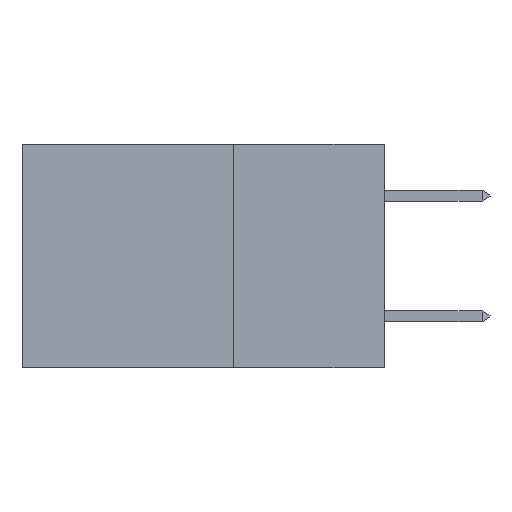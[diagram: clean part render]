
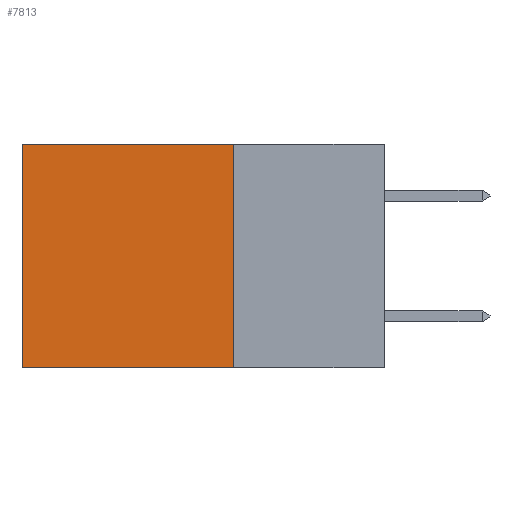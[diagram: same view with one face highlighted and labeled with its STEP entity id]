
A CAD part, left-side view. The second image highlights one B-rep face of the part: STEP entity #7813.
In plain terms, the highlighted planar face has unit normal (-1, 0, 0).
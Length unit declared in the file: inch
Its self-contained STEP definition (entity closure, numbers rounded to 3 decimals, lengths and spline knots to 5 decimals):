
#55 = VECTOR ( 'NONE', #8154, 39.37008 ) ;
#814 = EDGE_CURVE ( 'NONE', #9395, #15665, #13085, .T. ) ;
#1489 = ORIENTED_EDGE ( 'NONE', *, *, #814, .F. ) ;
#1760 = ORIENTED_EDGE ( 'NONE', *, *, #6386, .F. ) ;
#2906 = CARTESIAN_POINT ( 'NONE',  ( 0.2875, 0.25, 0. ) ) ;
#2936 = CARTESIAN_POINT ( 'NONE',  ( 0.2875, 0.25, 0. ) ) ;
#4235 = FACE_OUTER_BOUND ( 'NONE', #13283, .T. ) ;
#4544 = EDGE_CURVE ( 'NONE', #9395, #8620, #5394, .T. ) ;
#4994 = VERTEX_POINT ( 'NONE', #5558 ) ;
#5353 = CARTESIAN_POINT ( 'NONE',  ( 0.2875, 0.25, -0.37 ) ) ;
#5394 = LINE ( 'NONE', #11335, #7555 ) ;
#5558 = CARTESIAN_POINT ( 'NONE',  ( 0.2875, 0.6, -0.37 ) ) ;
#6169 = AXIS2_PLACEMENT_3D ( 'NONE', #2906, #8652, #14366 ) ;
#6386 = EDGE_CURVE ( 'NONE', #15665, #4994, #16621, .T. ) ;
#7189 = CARTESIAN_POINT ( 'NONE',  ( 0.2875, 0.6, 0. ) ) ;
#7555 = VECTOR ( 'NONE', #8414, 39.37008 ) ;
#7813 = ADVANCED_FACE ( 'NONE', ( #4235 ), #14451, .F. ) ;
#8154 = DIRECTION ( 'NONE',  ( 0., 0., -1. ) ) ;
#8414 = DIRECTION ( 'NONE',  ( 0., 1., 0. ) ) ;
#8620 = VERTEX_POINT ( 'NONE', #7189 ) ;
#8652 = DIRECTION ( 'NONE',  ( 1., 0., 0. ) ) ;
#9322 = CARTESIAN_POINT ( 'NONE',  ( 0.2875, 0.25, 0. ) ) ;
#9395 = VERTEX_POINT ( 'NONE', #9322 ) ;
#9489 = VECTOR ( 'NONE', #11600, 39.37008 ) ;
#11230 = ORIENTED_EDGE ( 'NONE', *, *, #4544, .T. ) ;
#11335 = CARTESIAN_POINT ( 'NONE',  ( 0.2875, 0.25, 0. ) ) ;
#11600 = DIRECTION ( 'NONE',  ( 0., 0., -1. ) ) ;
#12414 = DIRECTION ( 'NONE',  ( 0., 1., 0. ) ) ;
#13085 = LINE ( 'NONE', #2936, #9489 ) ;
#13283 = EDGE_LOOP ( 'NONE', ( #18202, #1760, #1489, #11230 ) ) ;
#14366 = DIRECTION ( 'NONE',  ( 0., 0., -1. ) ) ;
#14451 = PLANE ( 'NONE',  #6169 ) ;
#14499 = CARTESIAN_POINT ( 'NONE',  ( 0.2875, 0.25, -0.37 ) ) ;
#14999 = LINE ( 'NONE', #17991, #55 ) ;
#15665 = VERTEX_POINT ( 'NONE', #14499 ) ;
#16621 = LINE ( 'NONE', #5353, #17523 ) ;
#17334 = EDGE_CURVE ( 'NONE', #8620, #4994, #14999, .T. ) ;
#17523 = VECTOR ( 'NONE', #12414, 39.37008 ) ;
#17991 = CARTESIAN_POINT ( 'NONE',  ( 0.2875, 0.6, 0. ) ) ;
#18202 = ORIENTED_EDGE ( 'NONE', *, *, #17334, .T. ) ;
